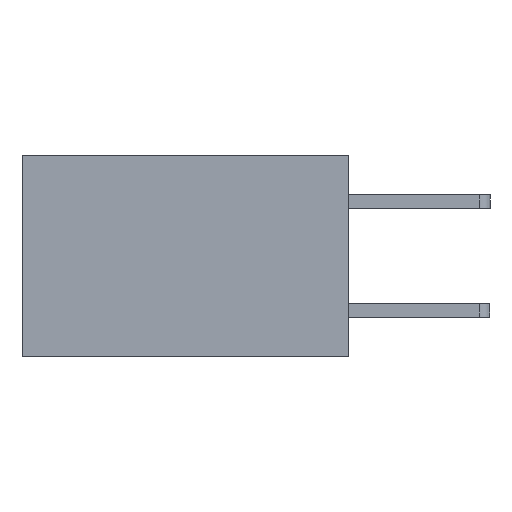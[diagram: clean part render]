
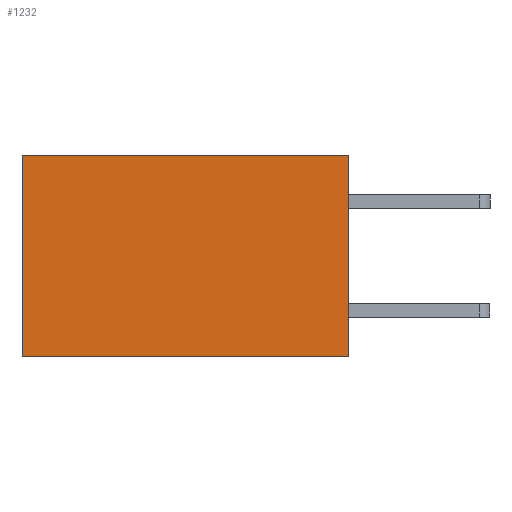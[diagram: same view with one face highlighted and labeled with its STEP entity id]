
A CAD part, left-side view. The second image highlights one B-rep face of the part: STEP entity #1232.
In plain terms, the highlighted planar face has unit normal (-1, 0, 0).
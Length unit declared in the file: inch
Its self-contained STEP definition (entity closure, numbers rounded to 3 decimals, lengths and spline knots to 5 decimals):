
#714 = VERTEX_POINT ( 'NONE', #978 ) ;
#856 = CARTESIAN_POINT ( 'NONE',  ( 0.298, 0., 0. ) ) ;
#978 = CARTESIAN_POINT ( 'NONE',  ( 0.298, 0.6, -0.37 ) ) ;
#1232 = ADVANCED_FACE ( 'NONE', ( #6511 ), #7436, .F. ) ;
#1726 = DIRECTION ( 'NONE',  ( 0., 0., -1. ) ) ;
#1893 = VERTEX_POINT ( 'NONE', #3733 ) ;
#2146 = EDGE_CURVE ( 'NONE', #1893, #714, #7246, .T. ) ;
#2179 = DIRECTION ( 'NONE',  ( 1., 0., 0. ) ) ;
#2245 = CARTESIAN_POINT ( 'NONE',  ( 0.298, 0.6, 0. ) ) ;
#3179 = CARTESIAN_POINT ( 'NONE',  ( 0.298, 0., -0.37 ) ) ;
#3301 = AXIS2_PLACEMENT_3D ( 'NONE', #7337, #2179, #1726 ) ;
#3733 = CARTESIAN_POINT ( 'NONE',  ( 0.298, 0., -0.37 ) ) ;
#4528 = DIRECTION ( 'NONE',  ( 0., 1., 0. ) ) ;
#4563 = VERTEX_POINT ( 'NONE', #856 ) ;
#5219 = ORIENTED_EDGE ( 'NONE', *, *, #8640, .F. ) ;
#5406 = VECTOR ( 'NONE', #7727, 39.37008 ) ;
#5609 = CARTESIAN_POINT ( 'NONE',  ( 0.298, 0., 0. ) ) ;
#5626 = DIRECTION ( 'NONE',  ( 0., 1., 0. ) ) ;
#5629 = LINE ( 'NONE', #5609, #5406 ) ;
#5790 = EDGE_CURVE ( 'NONE', #7621, #714, #9058, .T. ) ;
#6511 = FACE_OUTER_BOUND ( 'NONE', #10100, .T. ) ;
#7246 = LINE ( 'NONE', #3179, #7448 ) ;
#7315 = EDGE_CURVE ( 'NONE', #4563, #7621, #7500, .T. ) ;
#7337 = CARTESIAN_POINT ( 'NONE',  ( 0.298, 0., 0. ) ) ;
#7422 = ORIENTED_EDGE ( 'NONE', *, *, #5790, .T. ) ;
#7436 = PLANE ( 'NONE',  #3301 ) ;
#7448 = VECTOR ( 'NONE', #4528, 39.37008 ) ;
#7500 = LINE ( 'NONE', #9812, #9161 ) ;
#7621 = VERTEX_POINT ( 'NONE', #7947 ) ;
#7727 = DIRECTION ( 'NONE',  ( 0., 0., -1. ) ) ;
#7877 = ORIENTED_EDGE ( 'NONE', *, *, #2146, .F. ) ;
#7947 = CARTESIAN_POINT ( 'NONE',  ( 0.298, 0.6, 0. ) ) ;
#8512 = DIRECTION ( 'NONE',  ( 0., 0., -1. ) ) ;
#8640 = EDGE_CURVE ( 'NONE', #4563, #1893, #5629, .T. ) ;
#9058 = LINE ( 'NONE', #2245, #9283 ) ;
#9161 = VECTOR ( 'NONE', #5626, 39.37008 ) ;
#9283 = VECTOR ( 'NONE', #8512, 39.37008 ) ;
#9514 = ORIENTED_EDGE ( 'NONE', *, *, #7315, .T. ) ;
#9812 = CARTESIAN_POINT ( 'NONE',  ( 0.298, 0., 0. ) ) ;
#10100 = EDGE_LOOP ( 'NONE', ( #7422, #7877, #5219, #9514 ) ) ;
